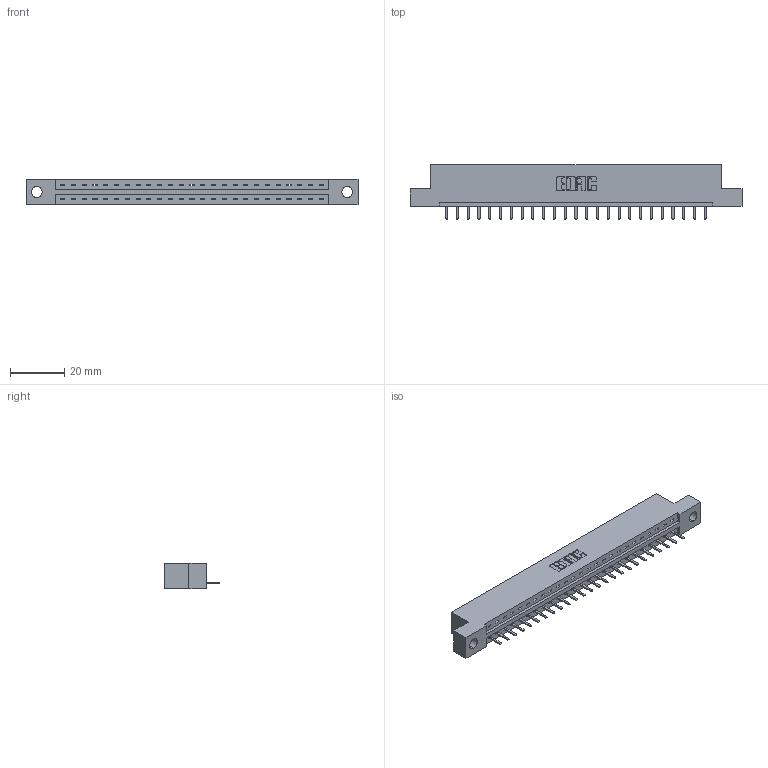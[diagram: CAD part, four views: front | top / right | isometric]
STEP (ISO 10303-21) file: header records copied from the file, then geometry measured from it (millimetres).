
FILE_DESCRIPTION (( 'STEP AP203' ), '1' );
FILE_NAME ('337-025-520-104.STEP', '2018-08-06T02:28:49', ( '' ), ( '' ), 'SwSTEP 2.0', 'SolidWorks 2016', '' );
FILE_SCHEMA (( 'CONFIG_CONTROL_DESIGN' ));
Length unit declared in the file: inch
Products named in the file (3): 337-025-520-104; 337 Part_Flush Mounting Lugs - 0.156 Dia-TH; 345-292-001_345-293-120
Assembly tree (26 placements, depth 2):
  337-025-520-104
    337 Part_Flush Mounting Lugs - 0.156 Dia-TH
    345-292-001_345-293-120  x25
Bounding box: 122.07 x 20.02 x 9.4 mm (x, y, z)
Volume: 12314.9 mm3; surface area: 12167.7 mm2
Topology: 26 solids, 26 shells, 1764 faces, 5211 edges, 3406 vertices
Faces by surface type: plane 1270, cylinder 494
Entity records: 20899 total; most frequent: CARTESIAN_POINT 3657, ORIENTED_EDGE 3606, DIRECTION 3101, EDGE_CURVE 1803, VECTOR 1671, LINE 1671, VERTEX_POINT 1198, AXIS2_PLACEMENT_3D 715
